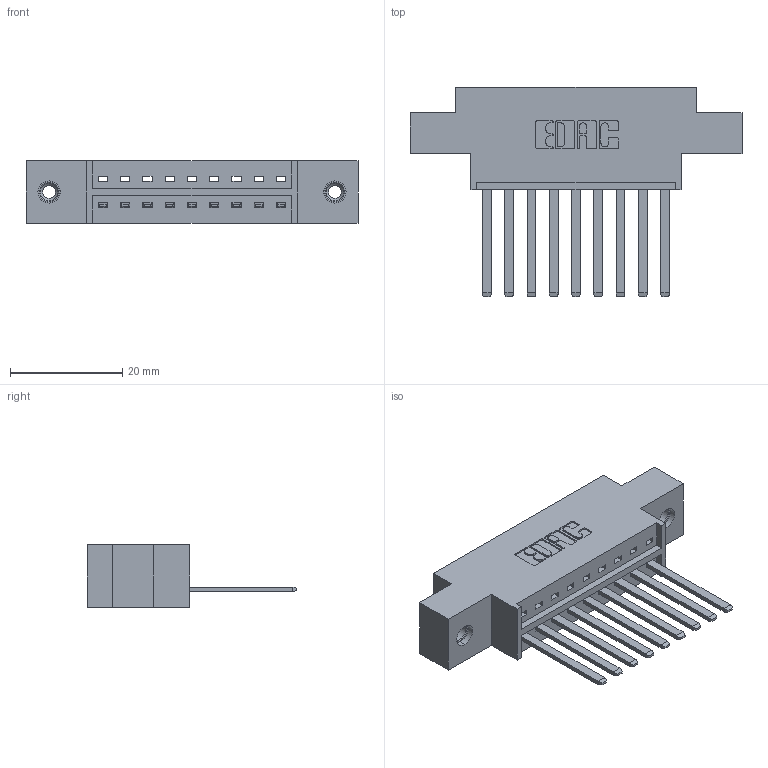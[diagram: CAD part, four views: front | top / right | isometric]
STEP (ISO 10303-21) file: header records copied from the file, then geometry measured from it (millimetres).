
FILE_DESCRIPTION (( 'STEP AP203' ), '1' );
FILE_NAME ('336-009-541-608.STEP', '2020-08-07T19:27:23', ( '' ), ( '' ), 'SwSTEP 2.0', 'SolidWorks 2020', '' );
FILE_SCHEMA (( 'CONFIG_CONTROL_DESIGN' ));
Length unit declared in the file: inch
Products named in the file (4): 345-250-001_345-250-003-102; 336-290-001_336-290-541; 336 Part_Offset - .156 Dia - TI; 336-009-541-608
Assembly tree (12 placements, depth 2):
  336-009-541-608
    336 Part_Offset - .156 Dia - TI
    336-290-001_336-290-541  x9
    345-250-001_345-250-003-102  x2
Bounding box: 59.05 x 37.34 x 11.1 mm (x, y, z)
Volume: 7643.8 mm3; surface area: 8008.2 mm2
Topology: 12 solids, 12 shells, 628 faces, 1845 edges, 1216 vertices
Faces by surface type: plane 412, cylinder 200, cone 12, torus 4
Entity records: 11995 total; most frequent: CARTESIAN_POINT 2151, ORIENTED_EDGE 1990, DIRECTION 1815, EDGE_CURVE 995, LINE 843, VECTOR 843, VERTEX_POINT 658, AXIS2_PLACEMENT_3D 486
